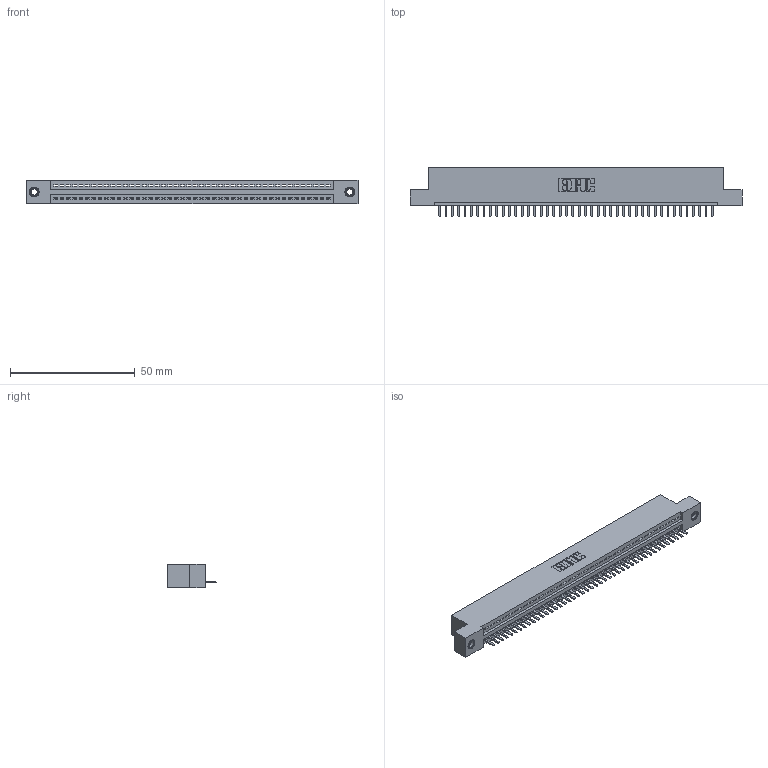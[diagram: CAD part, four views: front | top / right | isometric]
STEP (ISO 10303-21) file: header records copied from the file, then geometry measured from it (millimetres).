
FILE_DESCRIPTION (( 'STEP AP203' ), '1' );
FILE_NAME ('395-044-520-107.STEP', '2019-10-22T15:16:10', ( '' ), ( '' ), 'SwSTEP 2.0', 'SolidWorks 2016', '' );
FILE_SCHEMA (( 'CONFIG_CONTROL_DESIGN' ));
Length unit declared in the file: inch
Products named in the file (4): 345 Part_Flush Mounting Lugs - 0.156 Dia-TI; 395-044-520-107; 345-250-001_345-250-005-103; 345-292-001_345-293-120
Assembly tree (47 placements, depth 2):
  395-044-520-107
    345 Part_Flush Mounting Lugs - 0.156 Dia-TI
    345-292-001_345-293-120  x44
    345-250-001_345-250-005-103  x2
Bounding box: 132.97 x 19.68 x 9.4 mm (x, y, z)
Volume: 12505.8 mm3; surface area: 16264.8 mm2
Topology: 47 solids, 47 shells, 2914 faces, 8573 edges, 5590 vertices
Faces by surface type: plane 1960, cylinder 938, cone 12, torus 4
Entity records: 34146 total; most frequent: CARTESIAN_POINT 5907, ORIENTED_EDGE 5866, DIRECTION 5171, EDGE_CURVE 2933, LINE 2601, VECTOR 2601, VERTEX_POINT 1948, AXIS2_PLACEMENT_3D 1285
